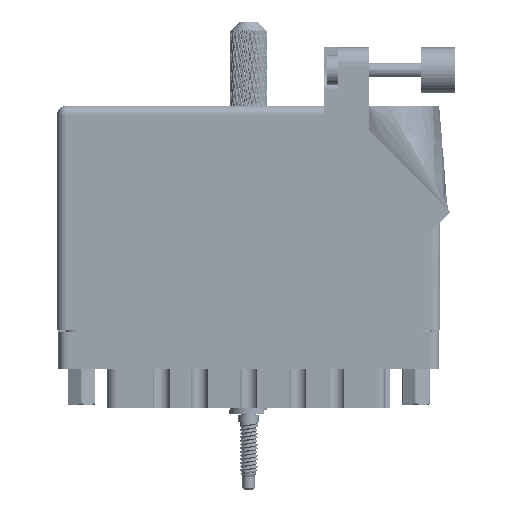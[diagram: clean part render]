
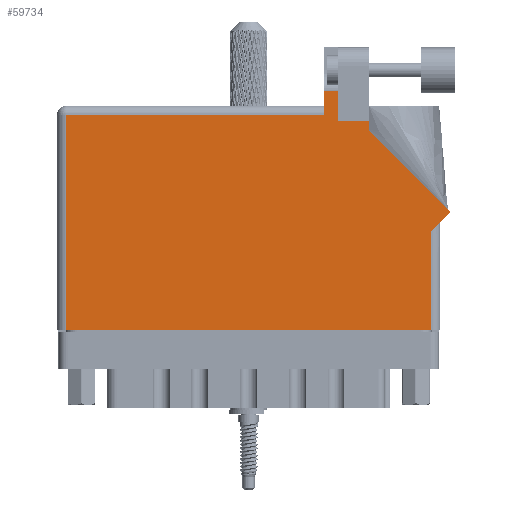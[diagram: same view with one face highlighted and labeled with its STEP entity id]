
A CAD part, front view. The second image highlights one B-rep face of the part: STEP entity #59734.
In plain terms, the highlighted face is planar.
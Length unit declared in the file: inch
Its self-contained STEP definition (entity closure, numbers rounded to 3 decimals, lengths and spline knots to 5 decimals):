
#179 = EDGE_LOOP ( 'NONE', ( #7449, #82351, #123292, #69517, #48578, #13253, #24966, #39845, #89457, #61462, #33852 ) ) ;
#890 = CARTESIAN_POINT ( 'NONE',  ( 0., 1.468, 0. ) ) ;
#3013 = CARTESIAN_POINT ( 'NONE',  ( 1.819, 1.6315, 0. ) ) ;
#5167 = VECTOR ( 'NONE', #63387, 39.37008 ) ;
#6678 = EDGE_CURVE ( 'NONE', #68660, #73694, #24927, .T. ) ;
#7449 = ORIENTED_EDGE ( 'NONE', *, *, #55917, .T. ) ;
#7941 = CARTESIAN_POINT ( 'NONE',  ( 1.913, 1.43, 0. ) ) ;
#9414 = VECTOR ( 'NONE', #122698, 39.37008 ) ;
#11805 = LINE ( 'NONE', #12988, #13413 ) ;
#12988 = CARTESIAN_POINT ( 'NONE',  ( 0.062, 0., 0. ) ) ;
#13253 = ORIENTED_EDGE ( 'NONE', *, *, #48660, .T. ) ;
#13413 = VECTOR ( 'NONE', #54071, 39.37008 ) ;
#15588 = DIRECTION ( 'NONE',  ( -1., 0., 0. ) ) ;
#18433 = VECTOR ( 'NONE', #105835, 39.37008 ) ;
#22684 = AXIS2_PLACEMENT_3D ( 'NONE', #124208, #64938, #15588 ) ;
#24695 = VECTOR ( 'NONE', #76396, 39.37008 ) ;
#24927 = LINE ( 'NONE', #43557, #9414 ) ;
#24966 = ORIENTED_EDGE ( 'NONE', *, *, #52579, .T. ) ;
#25101 = CARTESIAN_POINT ( 'NONE',  ( 2.55, 0.675, 0. ) ) ;
#25104 = PLANE ( 'NONE',  #22684 ) ;
#25532 = CARTESIAN_POINT ( 'NONE',  ( 1.819, 1.53, 0. ) ) ;
#25778 = CARTESIAN_POINT ( 'NONE',  ( 2.126, 1.43, 0. ) ) ;
#29219 = VERTEX_POINT ( 'NONE', #64061 ) ;
#31028 = CARTESIAN_POINT ( 'NONE',  ( 2.68271, 0.80771, 0. ) ) ;
#31304 = CARTESIAN_POINT ( 'NONE',  ( 1.913, 1.6315, 0. ) ) ;
#33055 = CARTESIAN_POINT ( 'NONE',  ( 2.24377, 1.6315, 0. ) ) ;
#33852 = ORIENTED_EDGE ( 'NONE', *, *, #83741, .T. ) ;
#37969 = EDGE_CURVE ( 'NONE', #94086, #90377, #50201, .T. ) ;
#38432 = FACE_OUTER_BOUND ( 'NONE', #179, .T. ) ;
#39845 = ORIENTED_EDGE ( 'NONE', *, *, #6678, .T. ) ;
#43274 = CARTESIAN_POINT ( 'NONE',  ( 2.55, 0.737, 0. ) ) ;
#43557 = CARTESIAN_POINT ( 'NONE',  ( 2.612, 0.737, 0. ) ) ;
#46125 = LINE ( 'NONE', #25532, #55464 ) ;
#46138 = DIRECTION ( 'NONE',  ( -1., 0., 0. ) ) ;
#47109 = VECTOR ( 'NONE', #119062, 39.37008 ) ;
#48578 = ORIENTED_EDGE ( 'NONE', *, *, #122967, .T. ) ;
#48660 = EDGE_CURVE ( 'NONE', #51625, #124164, #115383, .T. ) ;
#50201 = LINE ( 'NONE', #890, #47109 ) ;
#50935 = LINE ( 'NONE', #7941, #18433 ) ;
#51625 = VERTEX_POINT ( 'NONE', #110234 ) ;
#51744 = VECTOR ( 'NONE', #92268, 39.37008 ) ;
#52579 = EDGE_CURVE ( 'NONE', #124164, #68660, #115234, .T. ) ;
#53249 = LINE ( 'NONE', #33055, #5167 ) ;
#54071 = DIRECTION ( 'NONE',  ( 0., -1., 0. ) ) ;
#55464 = VECTOR ( 'NONE', #103911, 39.37008 ) ;
#55917 = EDGE_CURVE ( 'NONE', #99251, #90736, #50935, .T. ) ;
#56463 = CARTESIAN_POINT ( 'NONE',  ( 2.126, 1.36442, 0. ) ) ;
#59214 = VECTOR ( 'NONE', #60527, 39.37008 ) ;
#59734 = ADVANCED_FACE ( 'NONE', ( #38432 ), #25104, .F. ) ;
#60527 = DIRECTION ( 'NONE',  ( -0.707, 0.707, 0. ) ) ;
#61462 = ORIENTED_EDGE ( 'NONE', *, *, #72494, .T. ) ;
#62314 = EDGE_CURVE ( 'NONE', #73694, #29219, #90226, .T. ) ;
#63387 = DIRECTION ( 'NONE',  ( -1., 0., 0. ) ) ;
#64061 = CARTESIAN_POINT ( 'NONE',  ( 2.126, 1.36442, 0. ) ) ;
#64938 = DIRECTION ( 'NONE',  ( 0., 0., -1. ) ) ;
#68333 = LINE ( 'NONE', #25778, #91636 ) ;
#68660 = VERTEX_POINT ( 'NONE', #25101 ) ;
#69517 = ORIENTED_EDGE ( 'NONE', *, *, #37969, .T. ) ;
#69652 = CARTESIAN_POINT ( 'NONE',  ( 2.55, 0., 0. ) ) ;
#72494 = EDGE_CURVE ( 'NONE', #29219, #107900, #103742, .T. ) ;
#73694 = VERTEX_POINT ( 'NONE', #31028 ) ;
#76396 = DIRECTION ( 'NONE',  ( 0., 1., 0. ) ) ;
#82351 = ORIENTED_EDGE ( 'NONE', *, *, #112547, .T. ) ;
#83741 = EDGE_CURVE ( 'NONE', #107900, #99251, #68333, .T. ) ;
#89457 = ORIENTED_EDGE ( 'NONE', *, *, #62314, .T. ) ;
#90226 = LINE ( 'NONE', #99524, #59214 ) ;
#90377 = VERTEX_POINT ( 'NONE', #112067 ) ;
#90736 = VERTEX_POINT ( 'NONE', #31304 ) ;
#91636 = VECTOR ( 'NONE', #46138, 39.37008 ) ;
#92268 = DIRECTION ( 'NONE',  ( 0., 1., 0. ) ) ;
#93084 = DIRECTION ( 'NONE',  ( 1., 0., 0. ) ) ;
#94086 = VERTEX_POINT ( 'NONE', #123678 ) ;
#99251 = VERTEX_POINT ( 'NONE', #105769 ) ;
#99524 = CARTESIAN_POINT ( 'NONE',  ( 2.68271, 0.80771, 0. ) ) ;
#99549 = VERTEX_POINT ( 'NONE', #3013 ) ;
#101851 = EDGE_CURVE ( 'NONE', #99549, #94086, #46125, .T. ) ;
#103428 = CARTESIAN_POINT ( 'NONE',  ( 2.126, 1.43, 0. ) ) ;
#103742 = LINE ( 'NONE', #56463, #24695 ) ;
#103911 = DIRECTION ( 'NONE',  ( 0., -1., 0. ) ) ;
#105769 = CARTESIAN_POINT ( 'NONE',  ( 1.913, 1.43, 0. ) ) ;
#105835 = DIRECTION ( 'NONE',  ( 0., 1., 0. ) ) ;
#107900 = VERTEX_POINT ( 'NONE', #103428 ) ;
#110234 = CARTESIAN_POINT ( 'NONE',  ( 0.062, 0., 0. ) ) ;
#112067 = CARTESIAN_POINT ( 'NONE',  ( 0.062, 1.468, 0. ) ) ;
#112547 = EDGE_CURVE ( 'NONE', #90736, #99549, #53249, .T. ) ;
#113392 = CARTESIAN_POINT ( 'NONE',  ( 0., 0., 0. ) ) ;
#113914 = VECTOR ( 'NONE', #93084, 39.37008 ) ;
#115234 = LINE ( 'NONE', #43274, #51744 ) ;
#115383 = LINE ( 'NONE', #113392, #113914 ) ;
#119062 = DIRECTION ( 'NONE',  ( -1., 0., 0. ) ) ;
#122698 = DIRECTION ( 'NONE',  ( 0.707, 0.707, 0. ) ) ;
#122967 = EDGE_CURVE ( 'NONE', #90377, #51625, #11805, .T. ) ;
#123292 = ORIENTED_EDGE ( 'NONE', *, *, #101851, .T. ) ;
#123678 = CARTESIAN_POINT ( 'NONE',  ( 1.819, 1.468, 0. ) ) ;
#124164 = VERTEX_POINT ( 'NONE', #69652 ) ;
#124208 = CARTESIAN_POINT ( 'NONE',  ( 0., 1.53, 0. ) ) ;
